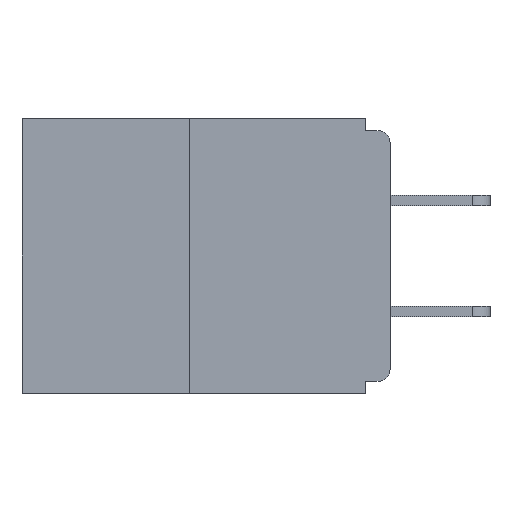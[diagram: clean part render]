
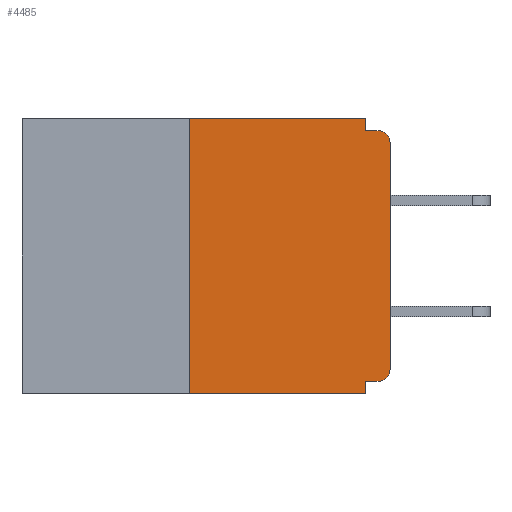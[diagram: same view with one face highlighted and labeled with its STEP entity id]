
A CAD part, left-side view. The second image highlights one B-rep face of the part: STEP entity #4485.
In plain terms, the highlighted planar face has unit normal (-1, 0, 0).
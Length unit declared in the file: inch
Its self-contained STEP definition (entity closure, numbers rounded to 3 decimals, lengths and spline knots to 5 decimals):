
#354 = ORIENTED_EDGE ( 'NONE', *, *, #797, .F. ) ;
#465 = EDGE_CURVE ( 'NONE', #7340, #7663, #6585, .T. ) ;
#500 = EDGE_CURVE ( 'NONE', #8953, #535, #1017, .T. ) ;
#518 = DIRECTION ( 'NONE',  ( 0., 0., -1. ) ) ;
#535 = VERTEX_POINT ( 'NONE', #6493 ) ;
#797 = EDGE_CURVE ( 'NONE', #8963, #9452, #8710, .T. ) ;
#816 = CARTESIAN_POINT ( 'NONE',  ( 0., 0.46, 0. ) ) ;
#845 = PLANE ( 'NONE',  #5931 ) ;
#1009 = VECTOR ( 'NONE', #10084, 39.37008 ) ;
#1017 = LINE ( 'NONE', #3688, #3061 ) ;
#1180 = LINE ( 'NONE', #5325, #1606 ) ;
#1334 = LINE ( 'NONE', #9523, #3791 ) ;
#1387 = CARTESIAN_POINT ( 'NONE',  ( 0., 0.031, -0.328 ) ) ;
#1606 = VECTOR ( 'NONE', #10570, 39.37008 ) ;
#1735 = VECTOR ( 'NONE', #7780, 39.37008 ) ;
#1764 = DIRECTION ( 'NONE',  ( 1., 0., 0. ) ) ;
#1835 = AXIS2_PLACEMENT_3D ( 'NONE', #5701, #3090, #518 ) ;
#1935 = LINE ( 'NONE', #10283, #6273 ) ;
#2070 = CIRCLE ( 'NONE', #10863, 0.015 ) ;
#2153 = VERTEX_POINT ( 'NONE', #1387 ) ;
#2180 = DIRECTION ( 'NONE',  ( 0., 0., 1. ) ) ;
#2312 = ORIENTED_EDGE ( 'NONE', *, *, #7460, .F. ) ;
#2411 = CARTESIAN_POINT ( 'NONE',  ( 0., 0., -0.313 ) ) ;
#2501 = CARTESIAN_POINT ( 'NONE',  ( 0., 0., 0. ) ) ;
#2541 = VECTOR ( 'NONE', #4804, 39.37008 ) ;
#2717 = CARTESIAN_POINT ( 'NONE',  ( 0., 0.25, 0. ) ) ;
#2728 = EDGE_CURVE ( 'NONE', #10628, #9370, #2070, .T. ) ;
#2760 = CARTESIAN_POINT ( 'NONE',  ( 0., 0.015, -0.313 ) ) ;
#3061 = VECTOR ( 'NONE', #7199, 39.37008 ) ;
#3090 = DIRECTION ( 'NONE',  ( -1., 0., 0. ) ) ;
#3199 = CARTESIAN_POINT ( 'NONE',  ( 0., 0.031, 0. ) ) ;
#3210 = EDGE_CURVE ( 'NONE', #9452, #7663, #1935, .T. ) ;
#3484 = ORIENTED_EDGE ( 'NONE', *, *, #11031, .T. ) ;
#3618 = LINE ( 'NONE', #9916, #2541 ) ;
#3688 = CARTESIAN_POINT ( 'NONE',  ( 0., 0.46, -0.343 ) ) ;
#3737 = CARTESIAN_POINT ( 'NONE',  ( 0., 0.25, 0. ) ) ;
#3791 = VECTOR ( 'NONE', #4028, 39.37008 ) ;
#4028 = DIRECTION ( 'NONE',  ( 0., 1., 0. ) ) ;
#4285 = ORIENTED_EDGE ( 'NONE', *, *, #9975, .F. ) ;
#4485 = ADVANCED_FACE ( 'NONE', ( #7042 ), #845, .F. ) ;
#4705 = LINE ( 'NONE', #2501, #1735 ) ;
#4804 = DIRECTION ( 'NONE',  ( 0., 0., -1. ) ) ;
#4838 = EDGE_CURVE ( 'NONE', #10628, #2153, #1334, .T. ) ;
#5131 = ORIENTED_EDGE ( 'NONE', *, *, #4838, .F. ) ;
#5293 = CARTESIAN_POINT ( 'NONE',  ( 0., 0.25, -0.343 ) ) ;
#5325 = CARTESIAN_POINT ( 'NONE',  ( 0., 0.46, 0. ) ) ;
#5701 = CARTESIAN_POINT ( 'NONE',  ( 0., 0.015, -0.03 ) ) ;
#5721 = LINE ( 'NONE', #3737, #8001 ) ;
#5931 = AXIS2_PLACEMENT_3D ( 'NONE', #816, #1764, #6016 ) ;
#6016 = DIRECTION ( 'NONE',  ( 0., 0., -1. ) ) ;
#6174 = CARTESIAN_POINT ( 'NONE',  ( 0., 0.031, 0. ) ) ;
#6273 = VECTOR ( 'NONE', #8640, 39.37008 ) ;
#6350 = ORIENTED_EDGE ( 'NONE', *, *, #500, .T. ) ;
#6493 = CARTESIAN_POINT ( 'NONE',  ( 0., 0.031, -0.343 ) ) ;
#6585 = CIRCLE ( 'NONE', #1835, 0.015 ) ;
#6735 = EDGE_LOOP ( 'NONE', ( #4285, #2312, #6350, #7622, #5131, #10371, #3484, #8758, #8679, #354 ) ) ;
#7042 = FACE_OUTER_BOUND ( 'NONE', #6735, .T. ) ;
#7199 = DIRECTION ( 'NONE',  ( 0., -1., 0. ) ) ;
#7340 = VERTEX_POINT ( 'NONE', #10496 ) ;
#7460 = EDGE_CURVE ( 'NONE', #8953, #8242, #5721, .T. ) ;
#7622 = ORIENTED_EDGE ( 'NONE', *, *, #10757, .F. ) ;
#7663 = VERTEX_POINT ( 'NONE', #9389 ) ;
#7780 = DIRECTION ( 'NONE',  ( 0., 0., 1. ) ) ;
#7941 = CARTESIAN_POINT ( 'NONE',  ( 0., 0.015, -0.328 ) ) ;
#8001 = VECTOR ( 'NONE', #2180, 39.37008 ) ;
#8242 = VERTEX_POINT ( 'NONE', #2717 ) ;
#8640 = DIRECTION ( 'NONE',  ( 0., -1., 0. ) ) ;
#8679 = ORIENTED_EDGE ( 'NONE', *, *, #3210, .F. ) ;
#8710 = LINE ( 'NONE', #3199, #1009 ) ;
#8758 = ORIENTED_EDGE ( 'NONE', *, *, #465, .T. ) ;
#8953 = VERTEX_POINT ( 'NONE', #5293 ) ;
#8963 = VERTEX_POINT ( 'NONE', #6174 ) ;
#9370 = VERTEX_POINT ( 'NONE', #2411 ) ;
#9389 = CARTESIAN_POINT ( 'NONE',  ( 0., 0.015, -0.015 ) ) ;
#9452 = VERTEX_POINT ( 'NONE', #10237 ) ;
#9523 = CARTESIAN_POINT ( 'NONE',  ( 0., 0., -0.328 ) ) ;
#9916 = CARTESIAN_POINT ( 'NONE',  ( 0., 0.031, -0.343 ) ) ;
#9975 = EDGE_CURVE ( 'NONE', #8242, #8963, #1180, .T. ) ;
#10084 = DIRECTION ( 'NONE',  ( 0., 0., -1. ) ) ;
#10237 = CARTESIAN_POINT ( 'NONE',  ( 0., 0.031, -0.015 ) ) ;
#10283 = CARTESIAN_POINT ( 'NONE',  ( 0., 0., -0.015 ) ) ;
#10371 = ORIENTED_EDGE ( 'NONE', *, *, #2728, .T. ) ;
#10496 = CARTESIAN_POINT ( 'NONE',  ( 0., 0., -0.03 ) ) ;
#10511 = DIRECTION ( 'NONE',  ( 0., 0., -1. ) ) ;
#10543 = DIRECTION ( 'NONE',  ( -1., 0., 0. ) ) ;
#10570 = DIRECTION ( 'NONE',  ( 0., -1., 0. ) ) ;
#10628 = VERTEX_POINT ( 'NONE', #7941 ) ;
#10757 = EDGE_CURVE ( 'NONE', #2153, #535, #3618, .T. ) ;
#10863 = AXIS2_PLACEMENT_3D ( 'NONE', #2760, #10543, #10511 ) ;
#11031 = EDGE_CURVE ( 'NONE', #9370, #7340, #4705, .T. ) ;
